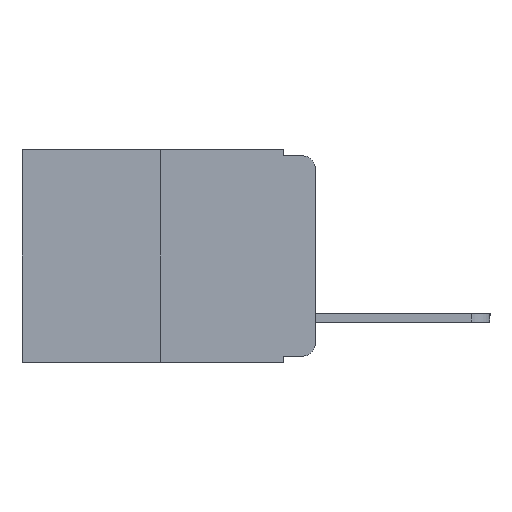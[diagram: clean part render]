
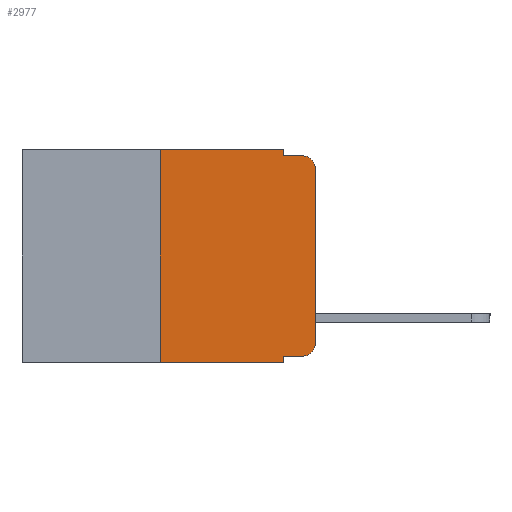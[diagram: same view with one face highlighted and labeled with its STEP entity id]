
A CAD part, left-side view. The second image highlights one B-rep face of the part: STEP entity #2977.
In plain terms, the highlighted planar face has unit normal (-1, 0, 0).
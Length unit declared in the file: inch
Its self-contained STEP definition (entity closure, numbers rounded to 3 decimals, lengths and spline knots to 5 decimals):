
#211 = CARTESIAN_POINT ( 'NONE',  ( 0., 0.051, 0. ) ) ;
#277 = CARTESIAN_POINT ( 'NONE',  ( 0., 0.02, -0.313 ) ) ;
#382 = DIRECTION ( 'NONE',  ( 0., 0., 1. ) ) ;
#429 = CARTESIAN_POINT ( 'NONE',  ( 0., 0.051, -0.01 ) ) ;
#549 = DIRECTION ( 'NONE',  ( 0., -1., 0. ) ) ;
#688 = CARTESIAN_POINT ( 'NONE',  ( 0., 0., 0. ) ) ;
#855 = LINE ( 'NONE', #7029, #3436 ) ;
#997 = EDGE_CURVE ( 'NONE', #1237, #1727, #4802, .T. ) ;
#1083 = ORIENTED_EDGE ( 'NONE', *, *, #8811, .T. ) ;
#1189 = ORIENTED_EDGE ( 'NONE', *, *, #3708, .T. ) ;
#1237 = VERTEX_POINT ( 'NONE', #8911 ) ;
#1432 = CIRCLE ( 'NONE', #3169, 0.02 ) ;
#1709 = ORIENTED_EDGE ( 'NONE', *, *, #8788, .F. ) ;
#1727 = VERTEX_POINT ( 'NONE', #2288 ) ;
#1903 = VECTOR ( 'NONE', #3619, 39.37008 ) ;
#1922 = VERTEX_POINT ( 'NONE', #211 ) ;
#2076 = CARTESIAN_POINT ( 'NONE',  ( 0., 0.02, -0.01 ) ) ;
#2097 = EDGE_LOOP ( 'NONE', ( #1189, #2180, #1709, #4702, #4917, #6359, #4890, #7501, #1083, #5189 ) ) ;
#2180 = ORIENTED_EDGE ( 'NONE', *, *, #9468, .T. ) ;
#2233 = DIRECTION ( 'NONE',  ( 0., 0., 1. ) ) ;
#2276 = EDGE_CURVE ( 'NONE', #1922, #8726, #9529, .T. ) ;
#2288 = CARTESIAN_POINT ( 'NONE',  ( 0., 0.051, -0.343 ) ) ;
#2391 = CARTESIAN_POINT ( 'NONE',  ( 0., 0.25, 0. ) ) ;
#2516 = EDGE_CURVE ( 'NONE', #2934, #1727, #8946, .T. ) ;
#2524 = LINE ( 'NONE', #2391, #11044 ) ;
#2934 = VERTEX_POINT ( 'NONE', #8325 ) ;
#2977 = ADVANCED_FACE ( 'NONE', ( #3159 ), #10094, .F. ) ;
#3141 = AXIS2_PLACEMENT_3D ( 'NONE', #277, #7009, #8109 ) ;
#3159 = FACE_OUTER_BOUND ( 'NONE', #2097, .T. ) ;
#3169 = AXIS2_PLACEMENT_3D ( 'NONE', #9425, #4609, #10162 ) ;
#3436 = VECTOR ( 'NONE', #7870, 39.37008 ) ;
#3619 = DIRECTION ( 'NONE',  ( 0., -1., 0. ) ) ;
#3708 = EDGE_CURVE ( 'NONE', #11145, #6872, #6583, .T. ) ;
#3723 = CARTESIAN_POINT ( 'NONE',  ( 0., 0.473, -0.343 ) ) ;
#3869 = CIRCLE ( 'NONE', #3141, 0.02 ) ;
#3930 = CARTESIAN_POINT ( 'NONE',  ( 0., 0.25, 0. ) ) ;
#4609 = DIRECTION ( 'NONE',  ( -1., 0., 0. ) ) ;
#4674 = VERTEX_POINT ( 'NONE', #3930 ) ;
#4702 = ORIENTED_EDGE ( 'NONE', *, *, #2276, .F. ) ;
#4802 = LINE ( 'NONE', #3723, #1903 ) ;
#4890 = ORIENTED_EDGE ( 'NONE', *, *, #997, .T. ) ;
#4917 = ORIENTED_EDGE ( 'NONE', *, *, #6807, .F. ) ;
#5089 = CARTESIAN_POINT ( 'NONE',  ( 0., 0.02, -0.333 ) ) ;
#5145 = CARTESIAN_POINT ( 'NONE',  ( 0., 0., -0.313 ) ) ;
#5189 = ORIENTED_EDGE ( 'NONE', *, *, #9494, .T. ) ;
#5518 = VERTEX_POINT ( 'NONE', #5089 ) ;
#6359 = ORIENTED_EDGE ( 'NONE', *, *, #11337, .F. ) ;
#6583 = LINE ( 'NONE', #688, #10959 ) ;
#6807 = EDGE_CURVE ( 'NONE', #4674, #1922, #11163, .T. ) ;
#6872 = VERTEX_POINT ( 'NONE', #7526 ) ;
#7009 = DIRECTION ( 'NONE',  ( -1., 0., 0. ) ) ;
#7029 = CARTESIAN_POINT ( 'NONE',  ( 0., 0.051, -0.333 ) ) ;
#7059 = DIRECTION ( 'NONE',  ( 0., 0., -1. ) ) ;
#7223 = VECTOR ( 'NONE', #7059, 39.37008 ) ;
#7501 = ORIENTED_EDGE ( 'NONE', *, *, #2516, .F. ) ;
#7526 = CARTESIAN_POINT ( 'NONE',  ( 0., 0., -0.03 ) ) ;
#7538 = CARTESIAN_POINT ( 'NONE',  ( 0., 0.051, 0. ) ) ;
#7562 = DIRECTION ( 'NONE',  ( 0., -1., 0. ) ) ;
#7831 = VERTEX_POINT ( 'NONE', #2076 ) ;
#7870 = DIRECTION ( 'NONE',  ( 0., -1., 0. ) ) ;
#8109 = DIRECTION ( 'NONE',  ( 0., 0., -1. ) ) ;
#8184 = LINE ( 'NONE', #9412, #9961 ) ;
#8325 = CARTESIAN_POINT ( 'NONE',  ( 0., 0.051, -0.333 ) ) ;
#8395 = DIRECTION ( 'NONE',  ( 0., 0., -1. ) ) ;
#8403 = CARTESIAN_POINT ( 'NONE',  ( 0., 0.473, 0. ) ) ;
#8489 = VECTOR ( 'NONE', #9082, 39.37008 ) ;
#8726 = VERTEX_POINT ( 'NONE', #429 ) ;
#8788 = EDGE_CURVE ( 'NONE', #8726, #7831, #8184, .T. ) ;
#8811 = EDGE_CURVE ( 'NONE', #2934, #5518, #855, .T. ) ;
#8911 = CARTESIAN_POINT ( 'NONE',  ( 0., 0.25, -0.343 ) ) ;
#8942 = VECTOR ( 'NONE', #7562, 39.37008 ) ;
#8946 = LINE ( 'NONE', #11316, #8489 ) ;
#9082 = DIRECTION ( 'NONE',  ( 0., 0., -1. ) ) ;
#9412 = CARTESIAN_POINT ( 'NONE',  ( 0., 0.051, -0.01 ) ) ;
#9425 = CARTESIAN_POINT ( 'NONE',  ( 0., 0.02, -0.03 ) ) ;
#9468 = EDGE_CURVE ( 'NONE', #6872, #7831, #1432, .T. ) ;
#9494 = EDGE_CURVE ( 'NONE', #5518, #11145, #3869, .T. ) ;
#9529 = LINE ( 'NONE', #7538, #7223 ) ;
#9824 = DIRECTION ( 'NONE',  ( 1., 0., 0. ) ) ;
#9961 = VECTOR ( 'NONE', #549, 39.37008 ) ;
#10094 = PLANE ( 'NONE',  #11196 ) ;
#10162 = DIRECTION ( 'NONE',  ( 0., 0., -1. ) ) ;
#10311 = CARTESIAN_POINT ( 'NONE',  ( 0., 0.473, 0. ) ) ;
#10959 = VECTOR ( 'NONE', #382, 39.37008 ) ;
#11044 = VECTOR ( 'NONE', #2233, 39.37008 ) ;
#11145 = VERTEX_POINT ( 'NONE', #5145 ) ;
#11163 = LINE ( 'NONE', #8403, #8942 ) ;
#11196 = AXIS2_PLACEMENT_3D ( 'NONE', #10311, #9824, #8395 ) ;
#11316 = CARTESIAN_POINT ( 'NONE',  ( 0., 0.051, 0. ) ) ;
#11337 = EDGE_CURVE ( 'NONE', #1237, #4674, #2524, .T. ) ;
